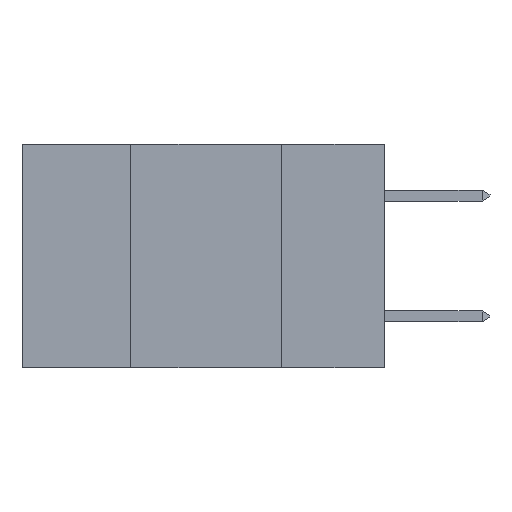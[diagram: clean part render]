
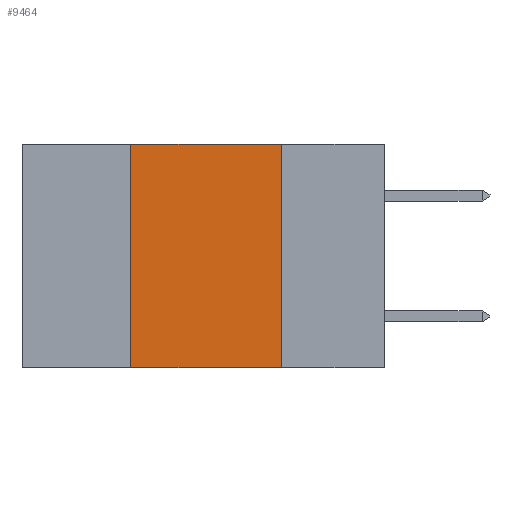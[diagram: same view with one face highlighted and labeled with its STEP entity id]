
A CAD part, left-side view. The second image highlights one B-rep face of the part: STEP entity #9464.
In plain terms, the highlighted planar face has unit normal (-1, 0, 0).
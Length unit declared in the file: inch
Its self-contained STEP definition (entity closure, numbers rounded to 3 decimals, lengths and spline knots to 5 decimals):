
#1045 = VECTOR ( 'NONE', #20450, 39.37008 ) ;
#1243 = VECTOR ( 'NONE', #7569, 39.37008 ) ;
#2726 = VERTEX_POINT ( 'NONE', #11503 ) ;
#2941 = VERTEX_POINT ( 'NONE', #12468 ) ;
#3358 = ORIENTED_EDGE ( 'NONE', *, *, #14846, .F. ) ;
#3486 = CARTESIAN_POINT ( 'NONE',  ( 0., 0.17, 0. ) ) ;
#4439 = EDGE_CURVE ( 'NONE', #2726, #2941, #8975, .T. ) ;
#4741 = DIRECTION ( 'NONE',  ( 0., 0., -1. ) ) ;
#6804 = DIRECTION ( 'NONE',  ( 0., 0., 1. ) ) ;
#7076 = ORIENTED_EDGE ( 'NONE', *, *, #9263, .T. ) ;
#7431 = LINE ( 'NONE', #20598, #18409 ) ;
#7569 = DIRECTION ( 'NONE',  ( 0., 0., -1. ) ) ;
#7899 = LINE ( 'NONE', #14373, #1045 ) ;
#8541 = CARTESIAN_POINT ( 'NONE',  ( 0., 0.6, 0. ) ) ;
#8975 = LINE ( 'NONE', #20183, #23555 ) ;
#9263 = EDGE_CURVE ( 'NONE', #2726, #16976, #7899, .T. ) ;
#9464 = ADVANCED_FACE ( 'NONE', ( #13806 ), #22003, .F. ) ;
#9545 = CARTESIAN_POINT ( 'NONE',  ( 0., 0.17, 0. ) ) ;
#9673 = DIRECTION ( 'NONE',  ( 0., -1., 0. ) ) ;
#11503 = CARTESIAN_POINT ( 'NONE',  ( 0., 0.42, -0.37 ) ) ;
#12468 = CARTESIAN_POINT ( 'NONE',  ( 0., 0.42, 0. ) ) ;
#13806 = FACE_OUTER_BOUND ( 'NONE', #22186, .T. ) ;
#14373 = CARTESIAN_POINT ( 'NONE',  ( 0., 0.6, -0.37 ) ) ;
#14846 = EDGE_CURVE ( 'NONE', #2941, #20563, #7431, .T. ) ;
#15991 = AXIS2_PLACEMENT_3D ( 'NONE', #8541, #19769, #4741 ) ;
#16976 = VERTEX_POINT ( 'NONE', #21784 ) ;
#17486 = ORIENTED_EDGE ( 'NONE', *, *, #4439, .F. ) ;
#18381 = EDGE_CURVE ( 'NONE', #20563, #16976, #19396, .T. ) ;
#18409 = VECTOR ( 'NONE', #9673, 39.37008 ) ;
#19396 = LINE ( 'NONE', #9545, #1243 ) ;
#19769 = DIRECTION ( 'NONE',  ( 1., 0., 0. ) ) ;
#20183 = CARTESIAN_POINT ( 'NONE',  ( 0., 0.42, 0. ) ) ;
#20450 = DIRECTION ( 'NONE',  ( 0., -1., 0. ) ) ;
#20520 = ORIENTED_EDGE ( 'NONE', *, *, #18381, .F. ) ;
#20563 = VERTEX_POINT ( 'NONE', #3486 ) ;
#20598 = CARTESIAN_POINT ( 'NONE',  ( 0., 0.6, 0. ) ) ;
#21784 = CARTESIAN_POINT ( 'NONE',  ( 0., 0.17, -0.37 ) ) ;
#22003 = PLANE ( 'NONE',  #15991 ) ;
#22186 = EDGE_LOOP ( 'NONE', ( #20520, #3358, #17486, #7076 ) ) ;
#23555 = VECTOR ( 'NONE', #6804, 39.37008 ) ;
